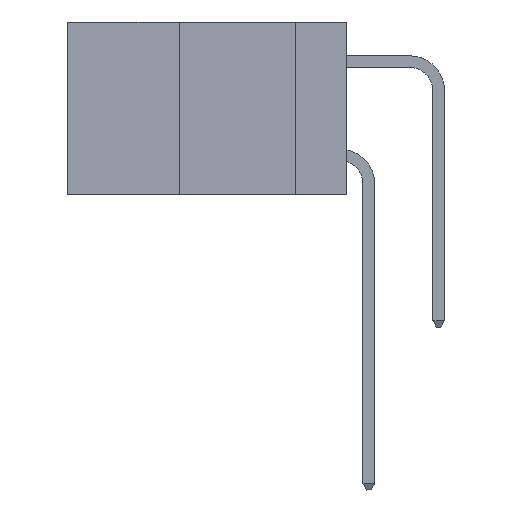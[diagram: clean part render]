
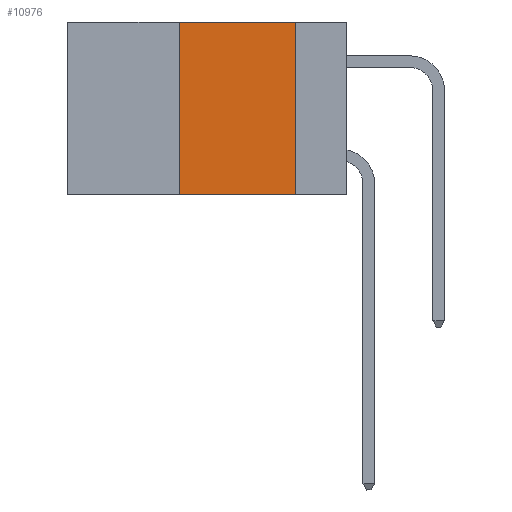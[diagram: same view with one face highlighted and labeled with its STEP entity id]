
A CAD part, left-side view. The second image highlights one B-rep face of the part: STEP entity #10976.
In plain terms, the highlighted planar face has unit normal (-1, 0, 0).
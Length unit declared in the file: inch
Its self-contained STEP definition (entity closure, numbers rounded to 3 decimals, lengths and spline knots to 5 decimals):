
#482 = CARTESIAN_POINT ( 'NONE',  ( 0., 0.36, 0. ) ) ;
#491 = DIRECTION ( 'NONE',  ( 1., 0., 0. ) ) ;
#541 = VECTOR ( 'NONE', #40854, 39.37008 ) ;
#2472 = EDGE_CURVE ( 'NONE', #6276, #11075, #25489, .T. ) ;
#3696 = DIRECTION ( 'NONE',  ( 0., 0., -1. ) ) ;
#3821 = DIRECTION ( 'NONE',  ( 0., 0., 1. ) ) ;
#4192 = LINE ( 'NONE', #482, #36132 ) ;
#5874 = ORIENTED_EDGE ( 'NONE', *, *, #2472, .F. ) ;
#6276 = VERTEX_POINT ( 'NONE', #10791 ) ;
#6987 = FACE_OUTER_BOUND ( 'NONE', #39845, .T. ) ;
#7674 = EDGE_CURVE ( 'NONE', #40066, #15090, #4192, .T. ) ;
#10527 = VECTOR ( 'NONE', #12852, 39.37008 ) ;
#10791 = CARTESIAN_POINT ( 'NONE',  ( 0., 0.11, 0. ) ) ;
#10976 = ADVANCED_FACE ( 'NONE', ( #6987 ), #32310, .F. ) ;
#11075 = VERTEX_POINT ( 'NONE', #29793 ) ;
#12852 = DIRECTION ( 'NONE',  ( 0., 0., -1. ) ) ;
#13224 = CARTESIAN_POINT ( 'NONE',  ( 0., 0.6, 0. ) ) ;
#15090 = VERTEX_POINT ( 'NONE', #20434 ) ;
#15674 = CARTESIAN_POINT ( 'NONE',  ( 0., 0.6, 0. ) ) ;
#20434 = CARTESIAN_POINT ( 'NONE',  ( 0., 0.36, 0. ) ) ;
#24764 = ORIENTED_EDGE ( 'NONE', *, *, #7674, .F. ) ;
#25489 = LINE ( 'NONE', #31515, #10527 ) ;
#28172 = CARTESIAN_POINT ( 'NONE',  ( 0., 0.6, -0.37 ) ) ;
#29295 = VECTOR ( 'NONE', #34564, 39.37008 ) ;
#29793 = CARTESIAN_POINT ( 'NONE',  ( 0., 0.11, -0.37 ) ) ;
#30490 = LINE ( 'NONE', #15674, #541 ) ;
#31515 = CARTESIAN_POINT ( 'NONE',  ( 0., 0.11, 0. ) ) ;
#32029 = AXIS2_PLACEMENT_3D ( 'NONE', #13224, #491, #3696 ) ;
#32310 = PLANE ( 'NONE',  #32029 ) ;
#34268 = LINE ( 'NONE', #28172, #29295 ) ;
#34564 = DIRECTION ( 'NONE',  ( 0., -1., 0. ) ) ;
#35357 = ORIENTED_EDGE ( 'NONE', *, *, #40247, .F. ) ;
#35414 = EDGE_CURVE ( 'NONE', #40066, #11075, #34268, .T. ) ;
#36132 = VECTOR ( 'NONE', #3821, 39.37008 ) ;
#37339 = ORIENTED_EDGE ( 'NONE', *, *, #35414, .T. ) ;
#39845 = EDGE_LOOP ( 'NONE', ( #5874, #35357, #24764, #37339 ) ) ;
#39909 = CARTESIAN_POINT ( 'NONE',  ( 0., 0.36, -0.37 ) ) ;
#40066 = VERTEX_POINT ( 'NONE', #39909 ) ;
#40247 = EDGE_CURVE ( 'NONE', #15090, #6276, #30490, .T. ) ;
#40854 = DIRECTION ( 'NONE',  ( 0., -1., 0. ) ) ;
